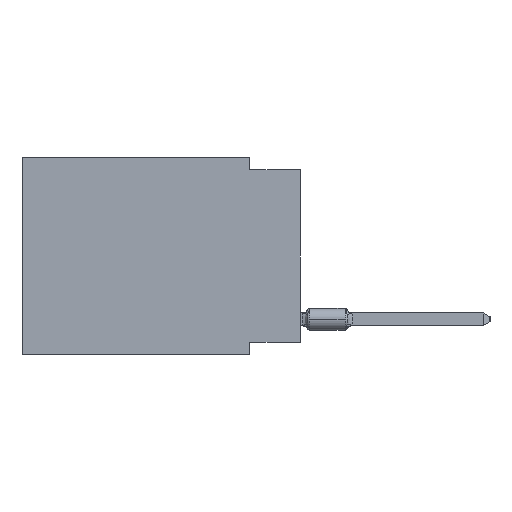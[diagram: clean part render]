
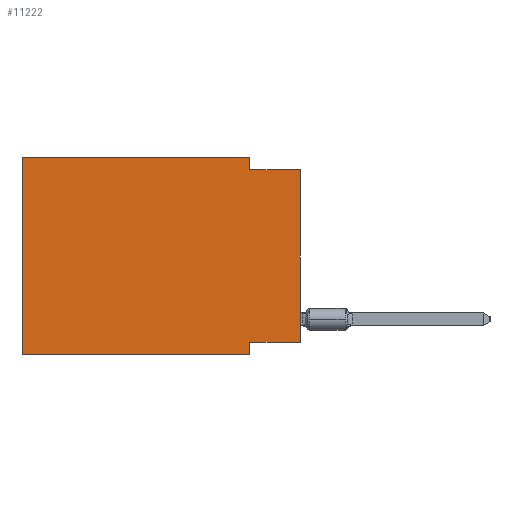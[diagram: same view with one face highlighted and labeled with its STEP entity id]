
A CAD part, left-side view. The second image highlights one B-rep face of the part: STEP entity #11222.
In plain terms, the highlighted planar face has unit normal (-1, 0, 0).
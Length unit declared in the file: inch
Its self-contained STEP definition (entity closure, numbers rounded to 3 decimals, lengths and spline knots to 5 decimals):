
#400 = EDGE_CURVE ( 'NONE', #40723, #42680, #21151, .T. ) ;
#510 = CARTESIAN_POINT ( 'NONE',  ( 0., 0., 0. ) ) ;
#523 = CARTESIAN_POINT ( 'NONE',  ( 0., 0., -0.025 ) ) ;
#1144 = CARTESIAN_POINT ( 'NONE',  ( 0., 0., -0.365 ) ) ;
#2488 = CARTESIAN_POINT ( 'NONE',  ( 0., 0., -0.025 ) ) ;
#3831 = DIRECTION ( 'NONE',  ( 0., 0., 1. ) ) ;
#4767 = ORIENTED_EDGE ( 'NONE', *, *, #7153, .F. ) ;
#4874 = DIRECTION ( 'NONE',  ( 0., -1., 0. ) ) ;
#5159 = VECTOR ( 'NONE', #58936, 39.37008 ) ;
#7019 = CARTESIAN_POINT ( 'NONE',  ( 0., 0.1, 0. ) ) ;
#7153 = EDGE_CURVE ( 'NONE', #42680, #12505, #56422, .T. ) ;
#8554 = CARTESIAN_POINT ( 'NONE',  ( 0., 0.55, 0. ) ) ;
#9341 = LINE ( 'NONE', #46796, #58062 ) ;
#11065 = CARTESIAN_POINT ( 'NONE',  ( 0., 0.55, 0. ) ) ;
#11154 = VERTEX_POINT ( 'NONE', #11065 ) ;
#11222 = ADVANCED_FACE ( 'NONE', ( #34072 ), #44823, .F. ) ;
#12221 = ORIENTED_EDGE ( 'NONE', *, *, #26461, .F. ) ;
#12505 = VERTEX_POINT ( 'NONE', #2488 ) ;
#14281 = ORIENTED_EDGE ( 'NONE', *, *, #55893, .F. ) ;
#15334 = EDGE_CURVE ( 'NONE', #18308, #12505, #42567, .T. ) ;
#18308 = VERTEX_POINT ( 'NONE', #1144 ) ;
#18848 = EDGE_CURVE ( 'NONE', #24908, #48071, #47322, .T. ) ;
#19199 = DIRECTION ( 'NONE',  ( 0., 0., 1. ) ) ;
#20628 = LINE ( 'NONE', #48620, #52593 ) ;
#21151 = LINE ( 'NONE', #21755, #54918 ) ;
#21399 = LINE ( 'NONE', #31554, #5159 ) ;
#21755 = CARTESIAN_POINT ( 'NONE',  ( 0., 0.1, 0. ) ) ;
#23378 = VECTOR ( 'NONE', #42870, 39.37008 ) ;
#24908 = VERTEX_POINT ( 'NONE', #39354 ) ;
#26461 = EDGE_CURVE ( 'NONE', #18308, #24908, #21399, .T. ) ;
#26515 = AXIS2_PLACEMENT_3D ( 'NONE', #54667, #34983, #44228 ) ;
#28745 = ORIENTED_EDGE ( 'NONE', *, *, #52340, .F. ) ;
#30583 = ORIENTED_EDGE ( 'NONE', *, *, #400, .F. ) ;
#31554 = CARTESIAN_POINT ( 'NONE',  ( 0., 0., -0.365 ) ) ;
#33761 = VECTOR ( 'NONE', #19199, 39.37008 ) ;
#34072 = FACE_OUTER_BOUND ( 'NONE', #55856, .T. ) ;
#34983 = DIRECTION ( 'NONE',  ( 1., 0., 0. ) ) ;
#35565 = VERTEX_POINT ( 'NONE', #58545 ) ;
#35599 = VECTOR ( 'NONE', #4874, 39.37008 ) ;
#36856 = CARTESIAN_POINT ( 'NONE',  ( 0., 0.1, -0.39 ) ) ;
#38881 = ORIENTED_EDGE ( 'NONE', *, *, #18848, .F. ) ;
#39070 = DIRECTION ( 'NONE',  ( 0., -1., 0. ) ) ;
#39354 = CARTESIAN_POINT ( 'NONE',  ( 0., 0.1, -0.365 ) ) ;
#40723 = VERTEX_POINT ( 'NONE', #7019 ) ;
#42013 = LINE ( 'NONE', #8554, #35599 ) ;
#42567 = LINE ( 'NONE', #510, #33761 ) ;
#42680 = VERTEX_POINT ( 'NONE', #44747 ) ;
#42870 = DIRECTION ( 'NONE',  ( 0., -1., 0. ) ) ;
#44228 = DIRECTION ( 'NONE',  ( 0., 0., -1. ) ) ;
#44638 = EDGE_CURVE ( 'NONE', #35565, #48071, #20628, .T. ) ;
#44747 = CARTESIAN_POINT ( 'NONE',  ( 0., 0.1, -0.025 ) ) ;
#44823 = PLANE ( 'NONE',  #26515 ) ;
#46796 = CARTESIAN_POINT ( 'NONE',  ( 0., 0.55, 0. ) ) ;
#47322 = LINE ( 'NONE', #51313, #59786 ) ;
#48071 = VERTEX_POINT ( 'NONE', #36856 ) ;
#48620 = CARTESIAN_POINT ( 'NONE',  ( 0., 0.55, -0.39 ) ) ;
#51313 = CARTESIAN_POINT ( 'NONE',  ( 0., 0.1, -0.39 ) ) ;
#52340 = EDGE_CURVE ( 'NONE', #35565, #11154, #9341, .T. ) ;
#52593 = VECTOR ( 'NONE', #39070, 39.37008 ) ;
#54665 = DIRECTION ( 'NONE',  ( 0., 0., -1. ) ) ;
#54667 = CARTESIAN_POINT ( 'NONE',  ( 0., 0.55, 0. ) ) ;
#54918 = VECTOR ( 'NONE', #54665, 39.37008 ) ;
#55856 = EDGE_LOOP ( 'NONE', ( #59916, #4767, #30583, #14281, #28745, #59320, #38881, #12221 ) ) ;
#55893 = EDGE_CURVE ( 'NONE', #11154, #40723, #42013, .T. ) ;
#56422 = LINE ( 'NONE', #523, #23378 ) ;
#56830 = DIRECTION ( 'NONE',  ( 0., 0., -1. ) ) ;
#58062 = VECTOR ( 'NONE', #3831, 39.37008 ) ;
#58545 = CARTESIAN_POINT ( 'NONE',  ( 0., 0.55, -0.39 ) ) ;
#58936 = DIRECTION ( 'NONE',  ( 0., 1., 0. ) ) ;
#59320 = ORIENTED_EDGE ( 'NONE', *, *, #44638, .T. ) ;
#59786 = VECTOR ( 'NONE', #56830, 39.37008 ) ;
#59916 = ORIENTED_EDGE ( 'NONE', *, *, #15334, .T. ) ;
